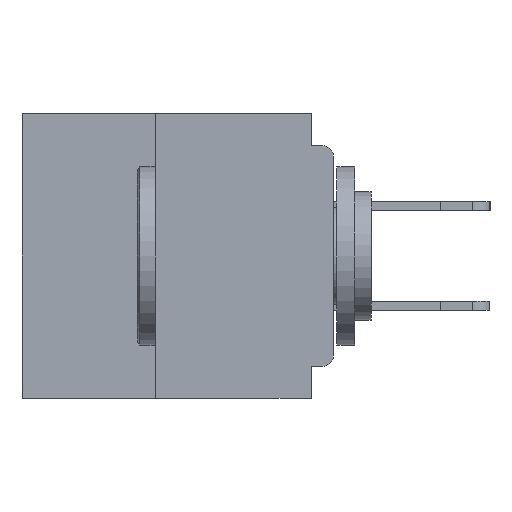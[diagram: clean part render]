
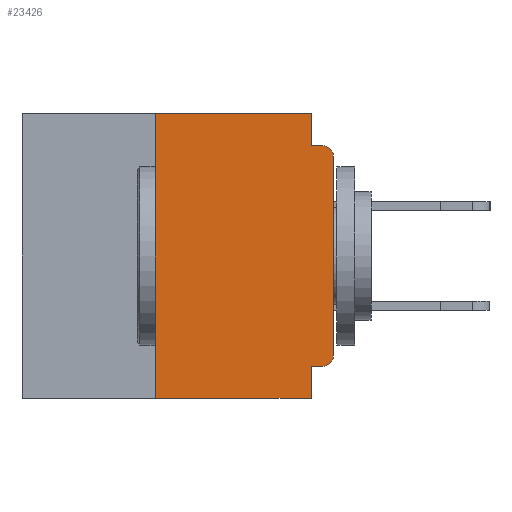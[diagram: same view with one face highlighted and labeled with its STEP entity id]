
A CAD part, left-side view. The second image highlights one B-rep face of the part: STEP entity #23426.
In plain terms, the highlighted planar face has unit normal (-1, 0, 0).
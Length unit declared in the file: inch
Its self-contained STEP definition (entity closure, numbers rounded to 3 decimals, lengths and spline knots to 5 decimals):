
#15 = ORIENTED_EDGE ( 'NONE', *, *, #36425, .F. ) ;
#692 = DIRECTION ( 'NONE',  ( 0., 0., 1. ) ) ;
#907 = ORIENTED_EDGE ( 'NONE', *, *, #42938, .T. ) ;
#918 = CARTESIAN_POINT ( 'NONE',  ( 0., 0.437, 0. ) ) ;
#1351 = CARTESIAN_POINT ( 'NONE',  ( 0., 0.015, -0.34 ) ) ;
#1503 = CARTESIAN_POINT ( 'NONE',  ( 0., 0., -0.06 ) ) ;
#2320 = CARTESIAN_POINT ( 'NONE',  ( 0., 0.437, -0.4 ) ) ;
#2529 = ORIENTED_EDGE ( 'NONE', *, *, #29167, .T. ) ;
#2762 = EDGE_CURVE ( 'NONE', #3239, #25593, #12169, .T. ) ;
#3239 = VERTEX_POINT ( 'NONE', #18812 ) ;
#4365 = DIRECTION ( 'NONE',  ( 0., 0., -1. ) ) ;
#4804 = DIRECTION ( 'NONE',  ( 0., 0., -1. ) ) ;
#4808 = ORIENTED_EDGE ( 'NONE', *, *, #28906, .F. ) ;
#5382 = VECTOR ( 'NONE', #6258, 39.37008 ) ;
#6258 = DIRECTION ( 'NONE',  ( 0., 1., 0. ) ) ;
#7011 = VERTEX_POINT ( 'NONE', #39872 ) ;
#7735 = CARTESIAN_POINT ( 'NONE',  ( 0., 0., 0. ) ) ;
#9532 = VECTOR ( 'NONE', #42950, 39.37008 ) ;
#9803 = ORIENTED_EDGE ( 'NONE', *, *, #2762, .F. ) ;
#9907 = LINE ( 'NONE', #7735, #35089 ) ;
#10329 = ORIENTED_EDGE ( 'NONE', *, *, #12844, .T. ) ;
#10914 = AXIS2_PLACEMENT_3D ( 'NONE', #918, #24936, #4365 ) ;
#11113 = PLANE ( 'NONE',  #10914 ) ;
#11444 = CARTESIAN_POINT ( 'NONE',  ( 0., 0.015, -0.06 ) ) ;
#11573 = CARTESIAN_POINT ( 'NONE',  ( 0., 0.031, 0. ) ) ;
#11758 = VECTOR ( 'NONE', #35514, 39.37008 ) ;
#12169 = LINE ( 'NONE', #30532, #37357 ) ;
#12374 = LINE ( 'NONE', #41414, #28479 ) ;
#12675 = CARTESIAN_POINT ( 'NONE',  ( 0., 0.015, -0.355 ) ) ;
#12844 = EDGE_CURVE ( 'NONE', #37168, #14868, #9907, .T. ) ;
#14459 = LINE ( 'NONE', #26842, #5382 ) ;
#14832 = DIRECTION ( 'NONE',  ( 0., 0., -1. ) ) ;
#14868 = VERTEX_POINT ( 'NONE', #1503 ) ;
#15207 = CARTESIAN_POINT ( 'NONE',  ( 0., 0., -0.34 ) ) ;
#15304 = CIRCLE ( 'NONE', #22297, 0.015 ) ;
#15336 = ORIENTED_EDGE ( 'NONE', *, *, #29427, .F. ) ;
#16251 = CARTESIAN_POINT ( 'NONE',  ( 0., 0.031, -0.355 ) ) ;
#18150 = EDGE_CURVE ( 'NONE', #32253, #29865, #25461, .T. ) ;
#18202 = VERTEX_POINT ( 'NONE', #16251 ) ;
#18812 = CARTESIAN_POINT ( 'NONE',  ( 0., 0.25, 0. ) ) ;
#18948 = EDGE_LOOP ( 'NONE', ( #10329, #907, #35490, #15, #9803, #4808, #32868, #34482, #15336, #2529 ) ) ;
#19457 = DIRECTION ( 'NONE',  ( 0., -1., 0. ) ) ;
#19597 = VERTEX_POINT ( 'NONE', #27735 ) ;
#19621 = CARTESIAN_POINT ( 'NONE',  ( 0., 0.25, -0.4 ) ) ;
#20916 = LINE ( 'NONE', #11573, #11758 ) ;
#22202 = CARTESIAN_POINT ( 'NONE',  ( 0., 0.031, -0.4 ) ) ;
#22297 = AXIS2_PLACEMENT_3D ( 'NONE', #11444, #35381, #14832 ) ;
#23426 = ADVANCED_FACE ( 'NONE', ( #33725 ), #11113, .F. ) ;
#23451 = CARTESIAN_POINT ( 'NONE',  ( 0., 0.031, 0. ) ) ;
#23912 = CARTESIAN_POINT ( 'NONE',  ( 0., 0.25, -0.4 ) ) ;
#24260 = EDGE_CURVE ( 'NONE', #7011, #19597, #29938, .T. ) ;
#24936 = DIRECTION ( 'NONE',  ( 1., 0., 0. ) ) ;
#25284 = CIRCLE ( 'NONE', #31413, 0.015 ) ;
#25378 = DIRECTION ( 'NONE',  ( -1., 0., 0. ) ) ;
#25461 = LINE ( 'NONE', #2320, #33435 ) ;
#25593 = VERTEX_POINT ( 'NONE', #23451 ) ;
#26842 = CARTESIAN_POINT ( 'NONE',  ( 0., 0., -0.355 ) ) ;
#26913 = VECTOR ( 'NONE', #27328, 39.37008 ) ;
#27328 = DIRECTION ( 'NONE',  ( 0., 0., 1. ) ) ;
#27735 = CARTESIAN_POINT ( 'NONE',  ( 0., 0.015, -0.045 ) ) ;
#27818 = DIRECTION ( 'NONE',  ( 0., 0., -1. ) ) ;
#27983 = LINE ( 'NONE', #23912, #26913 ) ;
#28479 = VECTOR ( 'NONE', #27818, 39.37008 ) ;
#28906 = EDGE_CURVE ( 'NONE', #32253, #3239, #27983, .T. ) ;
#29167 = EDGE_CURVE ( 'NONE', #38536, #37168, #25284, .T. ) ;
#29427 = EDGE_CURVE ( 'NONE', #38536, #18202, #14459, .T. ) ;
#29865 = VERTEX_POINT ( 'NONE', #22202 ) ;
#29938 = LINE ( 'NONE', #32642, #9532 ) ;
#30412 = DIRECTION ( 'NONE',  ( 0., -1., 0. ) ) ;
#30532 = CARTESIAN_POINT ( 'NONE',  ( 0., 0.437, 0. ) ) ;
#31413 = AXIS2_PLACEMENT_3D ( 'NONE', #1351, #25378, #4804 ) ;
#32253 = VERTEX_POINT ( 'NONE', #19621 ) ;
#32642 = CARTESIAN_POINT ( 'NONE',  ( 0., 0., -0.045 ) ) ;
#32868 = ORIENTED_EDGE ( 'NONE', *, *, #18150, .T. ) ;
#33435 = VECTOR ( 'NONE', #19457, 39.37008 ) ;
#33725 = FACE_OUTER_BOUND ( 'NONE', #18948, .T. ) ;
#34482 = ORIENTED_EDGE ( 'NONE', *, *, #40919, .F. ) ;
#35089 = VECTOR ( 'NONE', #692, 39.37008 ) ;
#35381 = DIRECTION ( 'NONE',  ( -1., 0., 0. ) ) ;
#35490 = ORIENTED_EDGE ( 'NONE', *, *, #24260, .F. ) ;
#35514 = DIRECTION ( 'NONE',  ( 0., 0., -1. ) ) ;
#36425 = EDGE_CURVE ( 'NONE', #25593, #7011, #20916, .T. ) ;
#37168 = VERTEX_POINT ( 'NONE', #15207 ) ;
#37357 = VECTOR ( 'NONE', #30412, 39.37008 ) ;
#38536 = VERTEX_POINT ( 'NONE', #12675 ) ;
#39872 = CARTESIAN_POINT ( 'NONE',  ( 0., 0.031, -0.045 ) ) ;
#40919 = EDGE_CURVE ( 'NONE', #18202, #29865, #12374, .T. ) ;
#41414 = CARTESIAN_POINT ( 'NONE',  ( 0., 0.031, -0.4 ) ) ;
#42938 = EDGE_CURVE ( 'NONE', #14868, #19597, #15304, .T. ) ;
#42950 = DIRECTION ( 'NONE',  ( 0., -1., 0. ) ) ;
